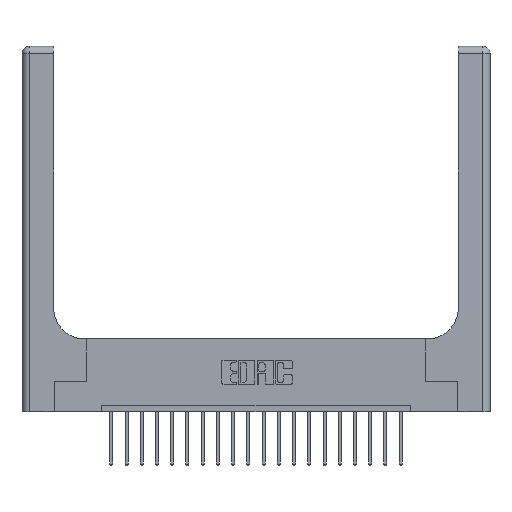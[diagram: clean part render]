
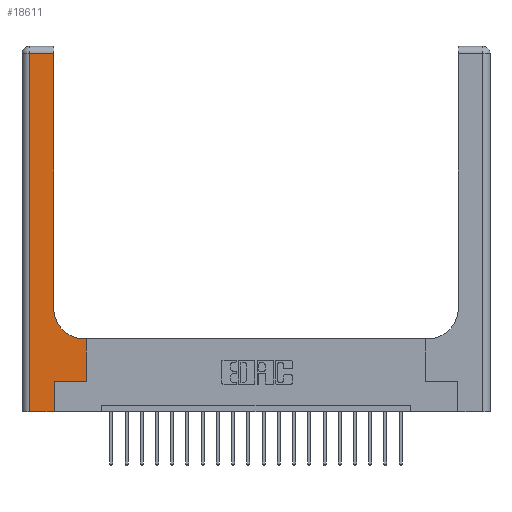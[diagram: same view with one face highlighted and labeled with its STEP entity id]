
A CAD part, top view. The second image highlights one B-rep face of the part: STEP entity #18611.
In plain terms, the highlighted planar face has unit normal (0, 0, 1).
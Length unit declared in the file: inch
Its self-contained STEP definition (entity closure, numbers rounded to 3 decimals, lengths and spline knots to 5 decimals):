
#290 = VECTOR ( 'NONE', #5189, 39.37008 ) ;
#452 = VERTEX_POINT ( 'NONE', #15083 ) ;
#902 = CARTESIAN_POINT ( 'NONE',  ( 0., 2.94, 0.37 ) ) ;
#1378 = CARTESIAN_POINT ( 'NONE',  ( 0.06, 3., 0.37 ) ) ;
#1747 = LINE ( 'NONE', #1904, #20368 ) ;
#1904 = CARTESIAN_POINT ( 'NONE',  ( 0.26, 3., 0.37 ) ) ;
#1946 = VECTOR ( 'NONE', #2300, 39.37008 ) ;
#2024 = EDGE_CURVE ( 'NONE', #3387, #10287, #12503, .T. ) ;
#2300 = DIRECTION ( 'NONE',  ( -1., 0., 0. ) ) ;
#2619 = DIRECTION ( 'NONE',  ( -1., 0., 0. ) ) ;
#2819 = ORIENTED_EDGE ( 'NONE', *, *, #4352, .T. ) ;
#3023 = EDGE_CURVE ( 'NONE', #19274, #8959, #5971, .T. ) ;
#3387 = VERTEX_POINT ( 'NONE', #19027 ) ;
#4097 = EDGE_LOOP ( 'NONE', ( #6935, #15336, #12659, #10057, #10359, #10680, #14837, #18902, #2819 ) ) ;
#4189 = DIRECTION ( 'NONE',  ( 0., 0., -1. ) ) ;
#4326 = DIRECTION ( 'NONE',  ( 0., -1., 0. ) ) ;
#4352 = EDGE_CURVE ( 'NONE', #18187, #16955, #20596, .T. ) ;
#4584 = LINE ( 'NONE', #902, #7069 ) ;
#4779 = LINE ( 'NONE', #15530, #6255 ) ;
#5043 = EDGE_CURVE ( 'NONE', #452, #19578, #19058, .T. ) ;
#5189 = DIRECTION ( 'NONE',  ( 0., 1., 0. ) ) ;
#5329 = CARTESIAN_POINT ( 'NONE',  ( 0.265, 0., 0.37 ) ) ;
#5630 = VECTOR ( 'NONE', #13138, 39.37008 ) ;
#5783 = DIRECTION ( 'NONE',  ( 0., 0., -1. ) ) ;
#5971 = LINE ( 'NONE', #5329, #290 ) ;
#5976 = CARTESIAN_POINT ( 'NONE',  ( 0.26, 0.85, 0.37 ) ) ;
#6255 = VECTOR ( 'NONE', #12377, 39.37008 ) ;
#6718 = AXIS2_PLACEMENT_3D ( 'NONE', #15223, #5783, #16835 ) ;
#6935 = ORIENTED_EDGE ( 'NONE', *, *, #17088, .T. ) ;
#7069 = VECTOR ( 'NONE', #2619, 39.37008 ) ;
#7398 = EDGE_CURVE ( 'NONE', #8959, #452, #4779, .T. ) ;
#8001 = AXIS2_PLACEMENT_3D ( 'NONE', #19844, #4189, #10327 ) ;
#8712 = CARTESIAN_POINT ( 'NONE',  ( 0.26, 0.6, 0.37 ) ) ;
#8753 = PLANE ( 'NONE',  #6718 ) ;
#8837 = LINE ( 'NONE', #8712, #1946 ) ;
#8959 = VERTEX_POINT ( 'NONE', #13118 ) ;
#9354 = DIRECTION ( 'NONE',  ( 1., 0., 0. ) ) ;
#9999 = EDGE_CURVE ( 'NONE', #13849, #3387, #4584, .T. ) ;
#10057 = ORIENTED_EDGE ( 'NONE', *, *, #15696, .T. ) ;
#10287 = VERTEX_POINT ( 'NONE', #15554 ) ;
#10292 = CARTESIAN_POINT ( 'NONE',  ( 0.528, 0.6, 0.37 ) ) ;
#10327 = DIRECTION ( 'NONE',  ( 1., 0., 0. ) ) ;
#10359 = ORIENTED_EDGE ( 'NONE', *, *, #3023, .T. ) ;
#10504 = VECTOR ( 'NONE', #4326, 39.37008 ) ;
#10680 = ORIENTED_EDGE ( 'NONE', *, *, #7398, .T. ) ;
#11540 = CARTESIAN_POINT ( 'NONE',  ( 0.528, 0.25, 0.37 ) ) ;
#11896 = VECTOR ( 'NONE', #9354, 39.37008 ) ;
#12377 = DIRECTION ( 'NONE',  ( 1., 0., 0. ) ) ;
#12503 = LINE ( 'NONE', #1378, #10504 ) ;
#12659 = ORIENTED_EDGE ( 'NONE', *, *, #2024, .T. ) ;
#12900 = LINE ( 'NONE', #17313, #11896 ) ;
#13118 = CARTESIAN_POINT ( 'NONE',  ( 0.265, 0.25, 0.37 ) ) ;
#13138 = DIRECTION ( 'NONE',  ( 0., 1., 0. ) ) ;
#13849 = VERTEX_POINT ( 'NONE', #15534 ) ;
#14099 = CARTESIAN_POINT ( 'NONE',  ( 0.51, 0.6, 0.37 ) ) ;
#14576 = DIRECTION ( 'NONE',  ( 0., 1., 0. ) ) ;
#14837 = ORIENTED_EDGE ( 'NONE', *, *, #5043, .T. ) ;
#15083 = CARTESIAN_POINT ( 'NONE',  ( 0.528, 0.25, 0.37 ) ) ;
#15223 = CARTESIAN_POINT ( 'NONE',  ( 0., 3., 0.37 ) ) ;
#15336 = ORIENTED_EDGE ( 'NONE', *, *, #9999, .T. ) ;
#15530 = CARTESIAN_POINT ( 'NONE',  ( 0.265, 0.25, 0.37 ) ) ;
#15534 = CARTESIAN_POINT ( 'NONE',  ( 0.26, 2.94, 0.37 ) ) ;
#15554 = CARTESIAN_POINT ( 'NONE',  ( 0.06, 0., 0.37 ) ) ;
#15696 = EDGE_CURVE ( 'NONE', #10287, #19274, #12900, .T. ) ;
#16835 = DIRECTION ( 'NONE',  ( -1., 0., 0. ) ) ;
#16955 = VERTEX_POINT ( 'NONE', #5976 ) ;
#17088 = EDGE_CURVE ( 'NONE', #16955, #13849, #1747, .T. ) ;
#17313 = CARTESIAN_POINT ( 'NONE',  ( 0., 0., 0.37 ) ) ;
#17906 = EDGE_CURVE ( 'NONE', #19578, #18187, #8837, .T. ) ;
#18187 = VERTEX_POINT ( 'NONE', #14099 ) ;
#18611 = ADVANCED_FACE ( 'NONE', ( #20317 ), #8753, .F. ) ;
#18895 = CARTESIAN_POINT ( 'NONE',  ( 0.265, 0., 0.37 ) ) ;
#18902 = ORIENTED_EDGE ( 'NONE', *, *, #17906, .T. ) ;
#19027 = CARTESIAN_POINT ( 'NONE',  ( 0.06, 2.94, 0.37 ) ) ;
#19058 = LINE ( 'NONE', #11540, #5630 ) ;
#19274 = VERTEX_POINT ( 'NONE', #18895 ) ;
#19578 = VERTEX_POINT ( 'NONE', #10292 ) ;
#19844 = CARTESIAN_POINT ( 'NONE',  ( 0.51, 0.85, 0.37 ) ) ;
#20317 = FACE_OUTER_BOUND ( 'NONE', #4097, .T. ) ;
#20368 = VECTOR ( 'NONE', #14576, 39.37008 ) ;
#20596 = CIRCLE ( 'NONE', #8001, 0.25 ) ;
